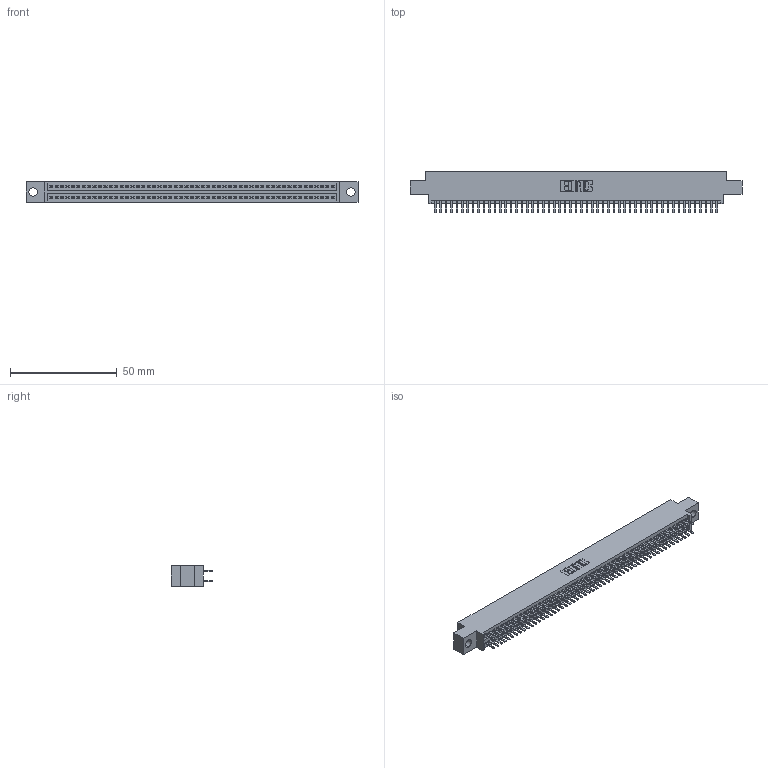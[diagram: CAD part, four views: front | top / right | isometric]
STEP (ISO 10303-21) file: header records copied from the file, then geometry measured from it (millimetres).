
FILE_DESCRIPTION (( 'STEP AP203' ), '1' );
FILE_NAME ('395-106-520-804.STEP', '2018-11-30T15:18:09', ( '' ), ( '' ), 'SwSTEP 2.0', 'SolidWorks 2016', '' );
FILE_SCHEMA (( 'CONFIG_CONTROL_DESIGN' ));
Length unit declared in the file: inch
Products named in the file (3): 345 Part_0.170 Offset - 0.156 Dia-TH; 395-106-520-804; 345-292-001_345-293-120
Assembly tree (107 placements, depth 2):
  395-106-520-804
    345 Part_0.170 Offset - 0.156 Dia-TH
    345-292-001_345-293-120  x106
Bounding box: 155.83 x 19.68 x 9.4 mm (x, y, z)
Volume: 14991.7 mm3; surface area: 22232.8 mm2
Topology: 107 solids, 107 shells, 5854 faces, 16995 edges, 11046 vertices
Faces by surface type: plane 3794, cylinder 2060
Entity records: 40353 total; most frequent: CARTESIAN_POINT 6768, ORIENTED_EDGE 6690, DIRECTION 5941, EDGE_CURVE 3345, LINE 2997, VECTOR 2997, VERTEX_POINT 2226, AXIS2_PLACEMENT_3D 1472
